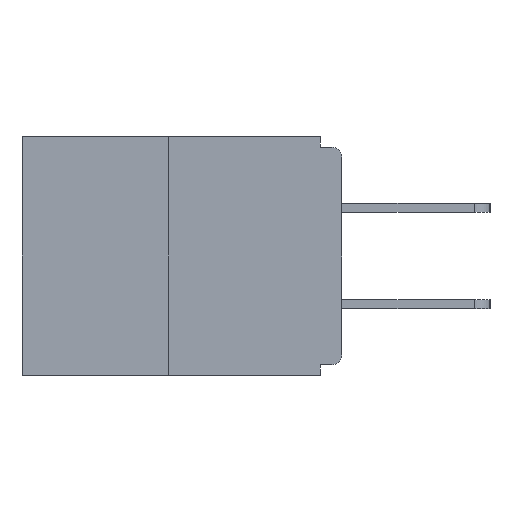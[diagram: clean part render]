
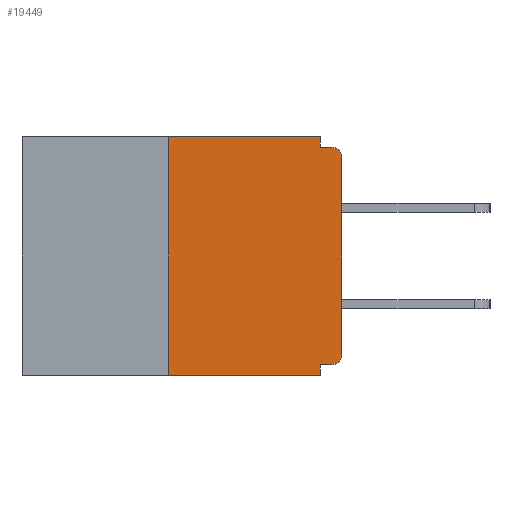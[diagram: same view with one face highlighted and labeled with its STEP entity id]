
A CAD part, left-side view. The second image highlights one B-rep face of the part: STEP entity #19449.
In plain terms, the highlighted planar face has unit normal (-1, 0, 0).
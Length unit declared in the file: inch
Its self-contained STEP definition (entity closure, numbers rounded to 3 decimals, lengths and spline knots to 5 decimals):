
#881 = VERTEX_POINT ( 'NONE', #2075 ) ;
#948 = LINE ( 'NONE', #13409, #16900 ) ;
#969 = VECTOR ( 'NONE', #20173, 39.37008 ) ;
#1124 = EDGE_CURVE ( 'NONE', #881, #6818, #12257, .T. ) ;
#1139 = ORIENTED_EDGE ( 'NONE', *, *, #18013, .T. ) ;
#1249 = CARTESIAN_POINT ( 'NONE',  ( 0., 0., -0.328 ) ) ;
#1270 = LINE ( 'NONE', #5818, #1790 ) ;
#1307 = AXIS2_PLACEMENT_3D ( 'NONE', #18091, #10033, #14819 ) ;
#1741 = EDGE_CURVE ( 'NONE', #7309, #6801, #9472, .T. ) ;
#1790 = VECTOR ( 'NONE', #18046, 39.37008 ) ;
#2075 = CARTESIAN_POINT ( 'NONE',  ( 0., 0.031, -0.015 ) ) ;
#2181 = DIRECTION ( 'NONE',  ( 0., 0., -1. ) ) ;
#2377 = EDGE_CURVE ( 'NONE', #6580, #17421, #3903, .T. ) ;
#2754 = CARTESIAN_POINT ( 'NONE',  ( 0., 0., -0.015 ) ) ;
#2832 = CARTESIAN_POINT ( 'NONE',  ( 0., 0.031, -0.343 ) ) ;
#3040 = CARTESIAN_POINT ( 'NONE',  ( 0., 0., 0. ) ) ;
#3215 = AXIS2_PLACEMENT_3D ( 'NONE', #20157, #9200, #4368 ) ;
#3294 = CARTESIAN_POINT ( 'NONE',  ( 0., 0.031, 0. ) ) ;
#3903 = LINE ( 'NONE', #6663, #16126 ) ;
#4368 = DIRECTION ( 'NONE',  ( 0., 0., -1. ) ) ;
#4874 = LINE ( 'NONE', #3040, #16095 ) ;
#5039 = CARTESIAN_POINT ( 'NONE',  ( 0., 0.015, -0.015 ) ) ;
#5150 = EDGE_CURVE ( 'NONE', #17421, #881, #8800, .T. ) ;
#5328 = CARTESIAN_POINT ( 'NONE',  ( 0., 0.031, 0. ) ) ;
#5385 = ORIENTED_EDGE ( 'NONE', *, *, #5150, .F. ) ;
#5664 = EDGE_CURVE ( 'NONE', #6801, #12562, #1270, .T. ) ;
#5818 = CARTESIAN_POINT ( 'NONE',  ( 0., 0.031, -0.343 ) ) ;
#5858 = DIRECTION ( 'NONE',  ( 0., -1., 0. ) ) ;
#6415 = ORIENTED_EDGE ( 'NONE', *, *, #1741, .F. ) ;
#6580 = VERTEX_POINT ( 'NONE', #15284 ) ;
#6663 = CARTESIAN_POINT ( 'NONE',  ( 0., 0.46, 0. ) ) ;
#6801 = VERTEX_POINT ( 'NONE', #9863 ) ;
#6818 = VERTEX_POINT ( 'NONE', #5039 ) ;
#7309 = VERTEX_POINT ( 'NONE', #17289 ) ;
#7408 = ORIENTED_EDGE ( 'NONE', *, *, #2377, .F. ) ;
#7839 = ORIENTED_EDGE ( 'NONE', *, *, #14617, .F. ) ;
#8013 = VECTOR ( 'NONE', #5858, 39.37008 ) ;
#8126 = CARTESIAN_POINT ( 'NONE',  ( 0., 0.25, -0.343 ) ) ;
#8345 = VECTOR ( 'NONE', #9556, 39.37008 ) ;
#8774 = CIRCLE ( 'NONE', #1307, 0.015 ) ;
#8800 = LINE ( 'NONE', #5328, #10036 ) ;
#9200 = DIRECTION ( 'NONE',  ( -1., 0., 0. ) ) ;
#9472 = LINE ( 'NONE', #1249, #969 ) ;
#9556 = DIRECTION ( 'NONE',  ( 0., 0., 1. ) ) ;
#9863 = CARTESIAN_POINT ( 'NONE',  ( 0., 0.031, -0.328 ) ) ;
#9932 = DIRECTION ( 'NONE',  ( 0., -1., 0. ) ) ;
#10033 = DIRECTION ( 'NONE',  ( -1., 0., 0. ) ) ;
#10036 = VECTOR ( 'NONE', #2181, 39.37008 ) ;
#10269 = VERTEX_POINT ( 'NONE', #8126 ) ;
#10395 = EDGE_LOOP ( 'NONE', ( #7408, #7839, #17874, #18525, #6415, #1139, #20062, #16935, #20494, #5385 ) ) ;
#10423 = CARTESIAN_POINT ( 'NONE',  ( 0., 0.46, 0. ) ) ;
#11212 = AXIS2_PLACEMENT_3D ( 'NONE', #10423, #11901, #15081 ) ;
#11602 = EDGE_CURVE ( 'NONE', #15265, #16576, #4874, .T. ) ;
#11901 = DIRECTION ( 'NONE',  ( 1., 0., 0. ) ) ;
#12257 = LINE ( 'NONE', #2754, #8013 ) ;
#12562 = VERTEX_POINT ( 'NONE', #2832 ) ;
#12606 = EDGE_CURVE ( 'NONE', #16576, #6818, #16793, .T. ) ;
#13156 = CARTESIAN_POINT ( 'NONE',  ( 0., 0., -0.03 ) ) ;
#13344 = DIRECTION ( 'NONE',  ( 0., -1., 0. ) ) ;
#13409 = CARTESIAN_POINT ( 'NONE',  ( 0., 0.46, -0.343 ) ) ;
#13681 = CARTESIAN_POINT ( 'NONE',  ( 0., 0., -0.313 ) ) ;
#13965 = LINE ( 'NONE', #17554, #8345 ) ;
#14617 = EDGE_CURVE ( 'NONE', #10269, #6580, #13965, .T. ) ;
#14819 = DIRECTION ( 'NONE',  ( 0., 0., -1. ) ) ;
#15081 = DIRECTION ( 'NONE',  ( 0., 0., -1. ) ) ;
#15265 = VERTEX_POINT ( 'NONE', #13681 ) ;
#15284 = CARTESIAN_POINT ( 'NONE',  ( 0., 0.25, 0. ) ) ;
#15666 = DIRECTION ( 'NONE',  ( 0., 0., 1. ) ) ;
#16095 = VECTOR ( 'NONE', #15666, 39.37008 ) ;
#16126 = VECTOR ( 'NONE', #9932, 39.37008 ) ;
#16576 = VERTEX_POINT ( 'NONE', #13156 ) ;
#16793 = CIRCLE ( 'NONE', #3215, 0.015 ) ;
#16900 = VECTOR ( 'NONE', #13344, 39.37008 ) ;
#16935 = ORIENTED_EDGE ( 'NONE', *, *, #12606, .T. ) ;
#17289 = CARTESIAN_POINT ( 'NONE',  ( 0., 0.015, -0.328 ) ) ;
#17421 = VERTEX_POINT ( 'NONE', #3294 ) ;
#17554 = CARTESIAN_POINT ( 'NONE',  ( 0., 0.25, 0. ) ) ;
#17874 = ORIENTED_EDGE ( 'NONE', *, *, #20116, .T. ) ;
#17907 = FACE_OUTER_BOUND ( 'NONE', #10395, .T. ) ;
#18013 = EDGE_CURVE ( 'NONE', #7309, #15265, #8774, .T. ) ;
#18046 = DIRECTION ( 'NONE',  ( 0., 0., -1. ) ) ;
#18091 = CARTESIAN_POINT ( 'NONE',  ( 0., 0.015, -0.313 ) ) ;
#18525 = ORIENTED_EDGE ( 'NONE', *, *, #5664, .F. ) ;
#19449 = ADVANCED_FACE ( 'NONE', ( #17907 ), #19915, .F. ) ;
#19915 = PLANE ( 'NONE',  #11212 ) ;
#20062 = ORIENTED_EDGE ( 'NONE', *, *, #11602, .T. ) ;
#20116 = EDGE_CURVE ( 'NONE', #10269, #12562, #948, .T. ) ;
#20157 = CARTESIAN_POINT ( 'NONE',  ( 0., 0.015, -0.03 ) ) ;
#20173 = DIRECTION ( 'NONE',  ( 0., 1., 0. ) ) ;
#20494 = ORIENTED_EDGE ( 'NONE', *, *, #1124, .F. ) ;
